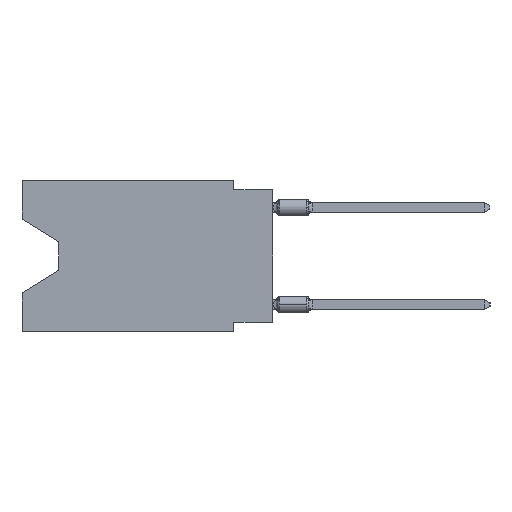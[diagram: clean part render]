
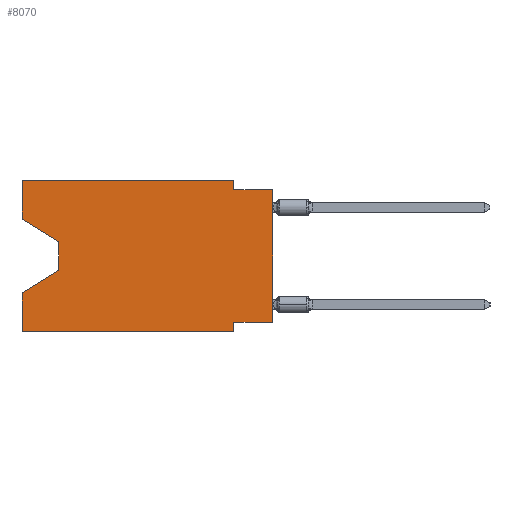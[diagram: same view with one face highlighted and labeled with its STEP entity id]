
A CAD part, left-side view. The second image highlights one B-rep face of the part: STEP entity #8070.
In plain terms, the highlighted planar face has unit normal (-1, 0, 0).
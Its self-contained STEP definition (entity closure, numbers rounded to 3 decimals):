
#73 = DIRECTION ( 'NONE',  ( 0., 0., -1. ) ) ;
#122 = DIRECTION ( 'NONE',  ( 0., 0., -1. ) ) ;
#211 = ORIENTED_EDGE ( 'NONE', *, *, #3094, .T. ) ;
#467 = LINE ( 'NONE', #3352, #25270 ) ;
#573 = DIRECTION ( 'NONE',  ( 0., -1., 0. ) ) ;
#1141 = ORIENTED_EDGE ( 'NONE', *, *, #6766, .F. ) ;
#1912 = ORIENTED_EDGE ( 'NONE', *, *, #2112, .T. ) ;
#2112 = EDGE_CURVE ( 'NONE', #31690, #7903, #12092, .T. ) ;
#2640 = DIRECTION ( 'NONE',  ( 0., 0., -1. ) ) ;
#2667 = AXIS2_PLACEMENT_3D ( 'NONE', #29645, #19871, #122 ) ;
#3094 = EDGE_CURVE ( 'NONE', #10028, #10473, #9327, .T. ) ;
#3352 = CARTESIAN_POINT ( 'NONE',  ( 0., 16.383, 0. ) ) ;
#3922 = CARTESIAN_POINT ( 'NONE',  ( 0., 0., -0.635 ) ) ;
#4972 = LINE ( 'NONE', #10952, #16133 ) ;
#5920 = ORIENTED_EDGE ( 'NONE', *, *, #6108, .F. ) ;
#6108 = EDGE_CURVE ( 'NONE', #10028, #35769, #467, .T. ) ;
#6208 = VECTOR ( 'NONE', #573, 1000. ) ;
#6428 = EDGE_CURVE ( 'NONE', #7903, #7220, #19479, .T. ) ;
#6458 = CARTESIAN_POINT ( 'NONE',  ( 0., 13.97, -5.893 ) ) ;
#6766 = EDGE_CURVE ( 'NONE', #36810, #11730, #16534, .T. ) ;
#7220 = VERTEX_POINT ( 'NONE', #6458 ) ;
#7882 = CARTESIAN_POINT ( 'NONE',  ( 0., 0., -0.635 ) ) ;
#7903 = VERTEX_POINT ( 'NONE', #36067 ) ;
#8070 = ADVANCED_FACE ( 'NONE', ( #13445 ), #39812, .F. ) ;
#8218 = ORIENTED_EDGE ( 'NONE', *, *, #41336, .F. ) ;
#9327 = LINE ( 'NONE', #9993, #37801 ) ;
#9993 = CARTESIAN_POINT ( 'NONE',  ( 0., 16.383, -9.906 ) ) ;
#10028 = VERTEX_POINT ( 'NONE', #31798 ) ;
#10405 = ORIENTED_EDGE ( 'NONE', *, *, #10823, .F. ) ;
#10473 = VERTEX_POINT ( 'NONE', #41922 ) ;
#10823 = EDGE_CURVE ( 'NONE', #11730, #32657, #23854, .T. ) ;
#10952 = CARTESIAN_POINT ( 'NONE',  ( 0., 16.383, 0. ) ) ;
#11026 = VECTOR ( 'NONE', #39429, 1000. ) ;
#11679 = DIRECTION ( 'NONE',  ( 0., 0., 1. ) ) ;
#11730 = VERTEX_POINT ( 'NONE', #18146 ) ;
#11736 = CARTESIAN_POINT ( 'NONE',  ( 0., 16.383, 0. ) ) ;
#12067 = CARTESIAN_POINT ( 'NONE',  ( 0., 2.54, -9.271 ) ) ;
#12092 = LINE ( 'NONE', #39340, #24628 ) ;
#12355 = ORIENTED_EDGE ( 'NONE', *, *, #6428, .T. ) ;
#12519 = VERTEX_POINT ( 'NONE', #34668 ) ;
#12698 = VERTEX_POINT ( 'NONE', #36621 ) ;
#13041 = LINE ( 'NONE', #36769, #11026 ) ;
#13445 = FACE_OUTER_BOUND ( 'NONE', #30634, .T. ) ;
#13994 = DIRECTION ( 'NONE',  ( 0., 0., 1. ) ) ;
#14346 = LINE ( 'NONE', #41621, #34222 ) ;
#15437 = CARTESIAN_POINT ( 'NONE',  ( 0., 16.383, -2.546 ) ) ;
#16133 = VECTOR ( 'NONE', #34894, 1000. ) ;
#16168 = CARTESIAN_POINT ( 'NONE',  ( 0., 13.97, -4.013 ) ) ;
#16534 = LINE ( 'NONE', #29634, #25379 ) ;
#18146 = CARTESIAN_POINT ( 'NONE',  ( 0., 2.54, -0.635 ) ) ;
#19479 = LINE ( 'NONE', #16168, #21006 ) ;
#19871 = DIRECTION ( 'NONE',  ( 1., 0., 0. ) ) ;
#20924 = VECTOR ( 'NONE', #33015, 1000. ) ;
#21006 = VECTOR ( 'NONE', #2640, 1000. ) ;
#21931 = DIRECTION ( 'NONE',  ( 0., 0., 1. ) ) ;
#22274 = DIRECTION ( 'NONE',  ( 0., -0.855, -0.519 ) ) ;
#22800 = LINE ( 'NONE', #39868, #20924 ) ;
#23854 = LINE ( 'NONE', #7882, #6208 ) ;
#24628 = VECTOR ( 'NONE', #22274, 1000. ) ;
#25270 = VECTOR ( 'NONE', #13994, 1000. ) ;
#25379 = VECTOR ( 'NONE', #36262, 1000. ) ;
#25625 = EDGE_CURVE ( 'NONE', #12519, #35561, #22800, .T. ) ;
#29032 = CARTESIAN_POINT ( 'NONE',  ( 0., 16.383, -7.36 ) ) ;
#29634 = CARTESIAN_POINT ( 'NONE',  ( 0., 2.54, 0. ) ) ;
#29645 = CARTESIAN_POINT ( 'NONE',  ( 0., 16.383, 0. ) ) ;
#30532 = ORIENTED_EDGE ( 'NONE', *, *, #39172, .T. ) ;
#30634 = EDGE_LOOP ( 'NONE', ( #1912, #12355, #30532, #5920, #211, #8218, #39597, #31818, #10405, #1141, #39838, #33046 ) ) ;
#31690 = VERTEX_POINT ( 'NONE', #15437 ) ;
#31706 = VECTOR ( 'NONE', #73, 1000. ) ;
#31798 = CARTESIAN_POINT ( 'NONE',  ( 0., 16.383, -9.906 ) ) ;
#31818 = ORIENTED_EDGE ( 'NONE', *, *, #32769, .T. ) ;
#32252 = CARTESIAN_POINT ( 'NONE',  ( 0., 2.54, 0. ) ) ;
#32458 = EDGE_CURVE ( 'NONE', #31690, #12698, #42094, .T. ) ;
#32657 = VERTEX_POINT ( 'NONE', #3922 ) ;
#32769 = EDGE_CURVE ( 'NONE', #12519, #32657, #14346, .T. ) ;
#33015 = DIRECTION ( 'NONE',  ( 0., 1., 0. ) ) ;
#33046 = ORIENTED_EDGE ( 'NONE', *, *, #32458, .F. ) ;
#33780 = LINE ( 'NONE', #36677, #31706 ) ;
#34222 = VECTOR ( 'NONE', #11679, 1000. ) ;
#34668 = CARTESIAN_POINT ( 'NONE',  ( 0., 0., -9.271 ) ) ;
#34894 = DIRECTION ( 'NONE',  ( 0., -1., 0. ) ) ;
#35561 = VERTEX_POINT ( 'NONE', #12067 ) ;
#35769 = VERTEX_POINT ( 'NONE', #29032 ) ;
#36067 = CARTESIAN_POINT ( 'NONE',  ( 0., 13.97, -4.013 ) ) ;
#36262 = DIRECTION ( 'NONE',  ( 0., 0., -1. ) ) ;
#36621 = CARTESIAN_POINT ( 'NONE',  ( 0., 16.383, 0. ) ) ;
#36677 = CARTESIAN_POINT ( 'NONE',  ( 0., 2.54, -9.906 ) ) ;
#36769 = CARTESIAN_POINT ( 'NONE',  ( 0., 13.97, -5.893 ) ) ;
#36810 = VERTEX_POINT ( 'NONE', #32252 ) ;
#37801 = VECTOR ( 'NONE', #43232, 1000. ) ;
#38449 = VECTOR ( 'NONE', #21931, 1000. ) ;
#39172 = EDGE_CURVE ( 'NONE', #7220, #35769, #13041, .T. ) ;
#39340 = CARTESIAN_POINT ( 'NONE',  ( 0., 16.383, -2.546 ) ) ;
#39429 = DIRECTION ( 'NONE',  ( 0., 0.855, -0.519 ) ) ;
#39597 = ORIENTED_EDGE ( 'NONE', *, *, #25625, .F. ) ;
#39812 = PLANE ( 'NONE',  #2667 ) ;
#39838 = ORIENTED_EDGE ( 'NONE', *, *, #43092, .F. ) ;
#39868 = CARTESIAN_POINT ( 'NONE',  ( 0., 0., -9.271 ) ) ;
#41336 = EDGE_CURVE ( 'NONE', #35561, #10473, #33780, .T. ) ;
#41621 = CARTESIAN_POINT ( 'NONE',  ( 0., 0., 0. ) ) ;
#41922 = CARTESIAN_POINT ( 'NONE',  ( 0., 2.54, -9.906 ) ) ;
#42094 = LINE ( 'NONE', #11736, #38449 ) ;
#43092 = EDGE_CURVE ( 'NONE', #12698, #36810, #4972, .T. ) ;
#43232 = DIRECTION ( 'NONE',  ( 0., -1., 0. ) ) ;
